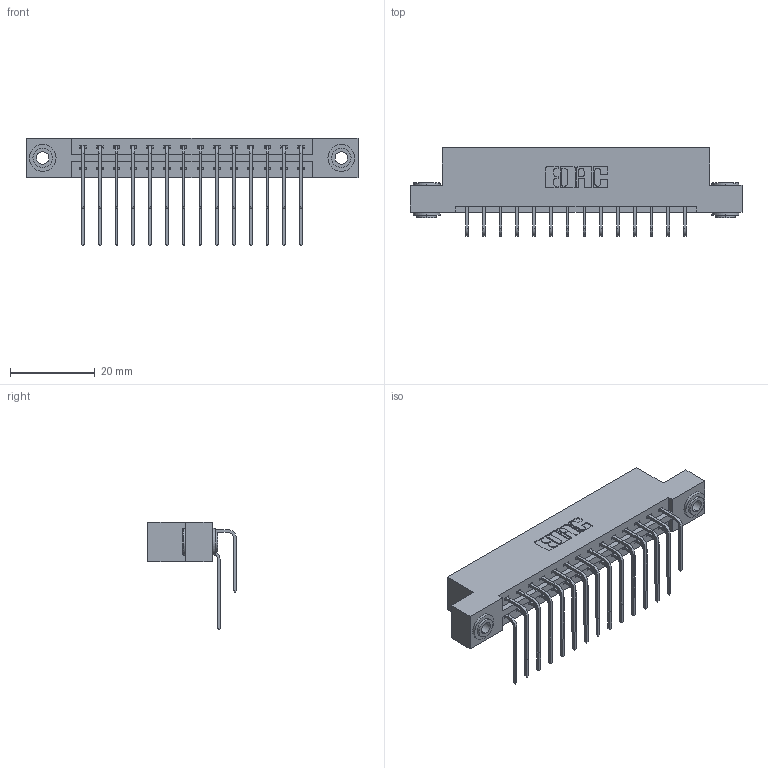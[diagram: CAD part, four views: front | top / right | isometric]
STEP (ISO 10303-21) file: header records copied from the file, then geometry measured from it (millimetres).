
FILE_DESCRIPTION (( 'STEP AP203' ), '1' );
FILE_NAME ('387-028-559-203.STEP', '2018-09-17T00:15:05', ( '' ), ( '' ), 'SwSTEP 2.0', 'SolidWorks 2016', '' );
FILE_SCHEMA (( 'CONFIG_CONTROL_DESIGN' ));
Length unit declared in the file: inch
Products named in the file (5): 345-292-001_559 Tail - 2; 345-250-002_345-250-002-102; 387-028-559-203; 337 Part_Flush Mounting Lugs - 0.156 Dia-TH; 345-292-001_558 559 Tail - 1
Assembly tree (31 placements, depth 2):
  387-028-559-203
    337 Part_Flush Mounting Lugs - 0.156 Dia-TH
    345-292-001_558 559 Tail - 1  x14
    345-292-001_559 Tail - 2  x14
    345-250-002_345-250-002-102  x2
Bounding box: 78.49 x 20.9 x 25.53 mm (x, y, z)
Volume: 8079.7 mm3; surface area: 9897.6 mm2
Topology: 31 solids, 31 shells, 1720 faces, 5063 edges, 3334 vertices
Faces by surface type: plane 1200, cylinder 512, cone 8
Entity records: 16910 total; most frequent: CARTESIAN_POINT 2892, ORIENTED_EDGE 2770, DIRECTION 2527, EDGE_CURVE 1385, VECTOR 1193, LINE 1193, VERTEX_POINT 918, AXIS2_PLACEMENT_3D 667
